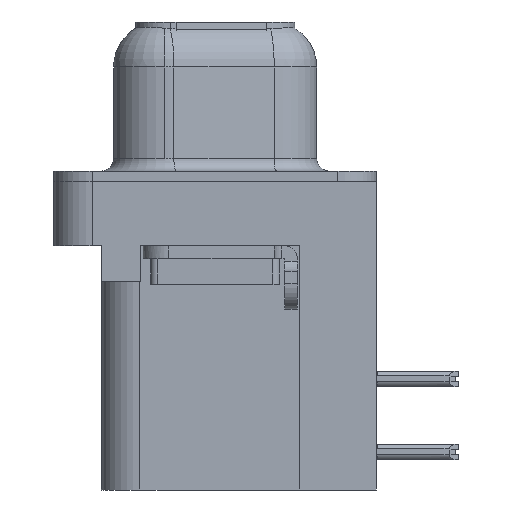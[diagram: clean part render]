
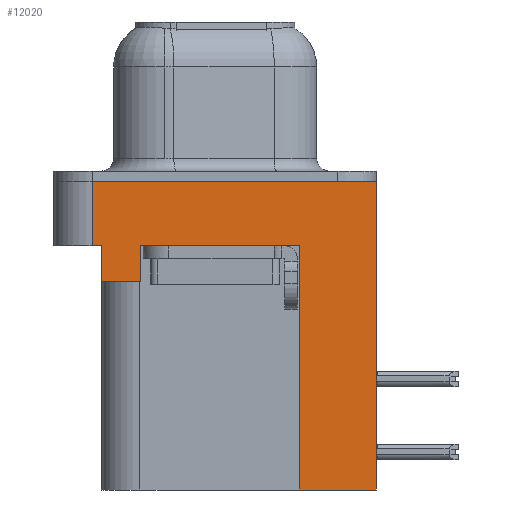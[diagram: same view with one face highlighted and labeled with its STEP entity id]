
A CAD part, left-side view. The second image highlights one B-rep face of the part: STEP entity #12020.
In plain terms, the highlighted planar face has unit normal (-1, 0, 0).
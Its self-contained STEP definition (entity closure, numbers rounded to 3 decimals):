
#141 = LINE ( 'NONE', #4457, #9080 ) ;
#143 = CARTESIAN_POINT ( 'NONE',  ( -2.91, -6.275, -12. ) ) ;
#186 = EDGE_CURVE ( 'NONE', #1064, #2829, #9140, .T. ) ;
#898 = CARTESIAN_POINT ( 'NONE',  ( -2.91, 4.775, -2.5 ) ) ;
#1064 = VERTEX_POINT ( 'NONE', #4011 ) ;
#1420 = CARTESIAN_POINT ( 'NONE',  ( -2.91, 4.425, -3.9 ) ) ;
#1840 = CARTESIAN_POINT ( 'NONE',  ( -2.91, 4.425, -2.5 ) ) ;
#2829 = VERTEX_POINT ( 'NONE', #13220 ) ;
#2948 = DIRECTION ( 'NONE',  ( 0., 0., 1. ) ) ;
#3089 = CARTESIAN_POINT ( 'NONE',  ( -2.91, -6.275, 0. ) ) ;
#3296 = VECTOR ( 'NONE', #19130, 1000. ) ;
#3628 = VECTOR ( 'NONE', #20773, 1000. ) ;
#3670 = ORIENTED_EDGE ( 'NONE', *, *, #15565, .F. ) ;
#3834 = DIRECTION ( 'NONE',  ( 0., 1., 0. ) ) ;
#3848 = CARTESIAN_POINT ( 'NONE',  ( -2.91, -3.295, -12. ) ) ;
#4011 = CARTESIAN_POINT ( 'NONE',  ( -2.91, 2.895, -3.9 ) ) ;
#4207 = LINE ( 'NONE', #10054, #13232 ) ;
#4291 = VERTEX_POINT ( 'NONE', #6107 ) ;
#4457 = CARTESIAN_POINT ( 'NONE',  ( -2.91, -6.275, 0. ) ) ;
#5781 = VECTOR ( 'NONE', #10627, 1000. ) ;
#5990 = EDGE_CURVE ( 'NONE', #15788, #20889, #21844, .T. ) ;
#6016 = DIRECTION ( 'NONE',  ( 0., 1., 0. ) ) ;
#6107 = CARTESIAN_POINT ( 'NONE',  ( -2.91, 2.895, -2.5 ) ) ;
#6413 = CARTESIAN_POINT ( 'NONE',  ( -2.91, 2.895, -3.9 ) ) ;
#6492 = EDGE_CURVE ( 'NONE', #10788, #13712, #4207, .T. ) ;
#6622 = AXIS2_PLACEMENT_3D ( 'NONE', #8035, #20778, #9815 ) ;
#6946 = VERTEX_POINT ( 'NONE', #3089 ) ;
#8035 = CARTESIAN_POINT ( 'NONE',  ( -2.91, -6.275, -2.5 ) ) ;
#8048 = DIRECTION ( 'NONE',  ( 0., -1., 0. ) ) ;
#8379 = EDGE_CURVE ( 'NONE', #2829, #13712, #16482, .T. ) ;
#9080 = VECTOR ( 'NONE', #8048, 1000. ) ;
#9140 = LINE ( 'NONE', #10991, #23173 ) ;
#9230 = VERTEX_POINT ( 'NONE', #22649 ) ;
#9815 = DIRECTION ( 'NONE',  ( 0., 0., 1. ) ) ;
#10054 = CARTESIAN_POINT ( 'NONE',  ( -2.91, -6.275, -2.5 ) ) ;
#10627 = DIRECTION ( 'NONE',  ( 0., 0., 1. ) ) ;
#10651 = EDGE_CURVE ( 'NONE', #10788, #22060, #13221, .T. ) ;
#10788 = VERTEX_POINT ( 'NONE', #23113 ) ;
#10991 = CARTESIAN_POINT ( 'NONE',  ( -2.91, 4.425, -3.9 ) ) ;
#11361 = VECTOR ( 'NONE', #2948, 1000. ) ;
#11423 = LINE ( 'NONE', #14219, #20583 ) ;
#11467 = ORIENTED_EDGE ( 'NONE', *, *, #21374, .T. ) ;
#11579 = VECTOR ( 'NONE', #19474, 1000. ) ;
#11619 = EDGE_CURVE ( 'NONE', #1064, #4291, #22053, .T. ) ;
#11896 = DIRECTION ( 'NONE',  ( 0., -1., 0. ) ) ;
#12020 = ADVANCED_FACE ( 'NONE', ( #15164 ), #15261, .T. ) ;
#13220 = CARTESIAN_POINT ( 'NONE',  ( -2.91, 4.425, -3.9 ) ) ;
#13221 = LINE ( 'NONE', #898, #3628 ) ;
#13232 = VECTOR ( 'NONE', #11896, 1000. ) ;
#13712 = VERTEX_POINT ( 'NONE', #1840 ) ;
#14219 = CARTESIAN_POINT ( 'NONE',  ( -2.91, -6.275, -2.5 ) ) ;
#14888 = ORIENTED_EDGE ( 'NONE', *, *, #5990, .F. ) ;
#15164 = FACE_OUTER_BOUND ( 'NONE', #23243, .T. ) ;
#15261 = PLANE ( 'NONE',  #6622 ) ;
#15565 = EDGE_CURVE ( 'NONE', #20889, #9230, #21095, .T. ) ;
#15788 = VERTEX_POINT ( 'NONE', #143 ) ;
#16038 = DIRECTION ( 'NONE',  ( 0., -1., 0. ) ) ;
#16482 = LINE ( 'NONE', #1420, #11579 ) ;
#17211 = ORIENTED_EDGE ( 'NONE', *, *, #186, .F. ) ;
#17471 = CARTESIAN_POINT ( 'NONE',  ( -2.91, -3.295, -12. ) ) ;
#18070 = ORIENTED_EDGE ( 'NONE', *, *, #23359, .F. ) ;
#19130 = DIRECTION ( 'NONE',  ( 0., 0., 1. ) ) ;
#19425 = ORIENTED_EDGE ( 'NONE', *, *, #20341, .T. ) ;
#19474 = DIRECTION ( 'NONE',  ( 0., 0., 1. ) ) ;
#19602 = ORIENTED_EDGE ( 'NONE', *, *, #11619, .T. ) ;
#19742 = CARTESIAN_POINT ( 'NONE',  ( -2.91, -6.275, -2.5 ) ) ;
#20263 = LINE ( 'NONE', #19742, #5781 ) ;
#20341 = EDGE_CURVE ( 'NONE', #4291, #9230, #11423, .T. ) ;
#20378 = ORIENTED_EDGE ( 'NONE', *, *, #10651, .F. ) ;
#20583 = VECTOR ( 'NONE', #16038, 1000. ) ;
#20773 = DIRECTION ( 'NONE',  ( 0., 0., 1. ) ) ;
#20778 = DIRECTION ( 'NONE',  ( -1., 0., 0. ) ) ;
#20889 = VERTEX_POINT ( 'NONE', #22923 ) ;
#21095 = LINE ( 'NONE', #17471, #11361 ) ;
#21374 = EDGE_CURVE ( 'NONE', #15788, #6946, #20263, .T. ) ;
#21422 = ORIENTED_EDGE ( 'NONE', *, *, #6492, .T. ) ;
#21844 = LINE ( 'NONE', #3848, #22415 ) ;
#22053 = LINE ( 'NONE', #6413, #3296 ) ;
#22060 = VERTEX_POINT ( 'NONE', #23481 ) ;
#22289 = ORIENTED_EDGE ( 'NONE', *, *, #8379, .F. ) ;
#22415 = VECTOR ( 'NONE', #3834, 1000. ) ;
#22649 = CARTESIAN_POINT ( 'NONE',  ( -2.91, -3.295, -2.5 ) ) ;
#22923 = CARTESIAN_POINT ( 'NONE',  ( -2.91, -3.295, -12. ) ) ;
#23113 = CARTESIAN_POINT ( 'NONE',  ( -2.91, 4.775, -2.5 ) ) ;
#23173 = VECTOR ( 'NONE', #6016, 1000. ) ;
#23243 = EDGE_LOOP ( 'NONE', ( #18070, #20378, #21422, #22289, #17211, #19602, #19425, #3670, #14888, #11467 ) ) ;
#23359 = EDGE_CURVE ( 'NONE', #22060, #6946, #141, .T. ) ;
#23481 = CARTESIAN_POINT ( 'NONE',  ( -2.91, 4.775, 0. ) ) ;
